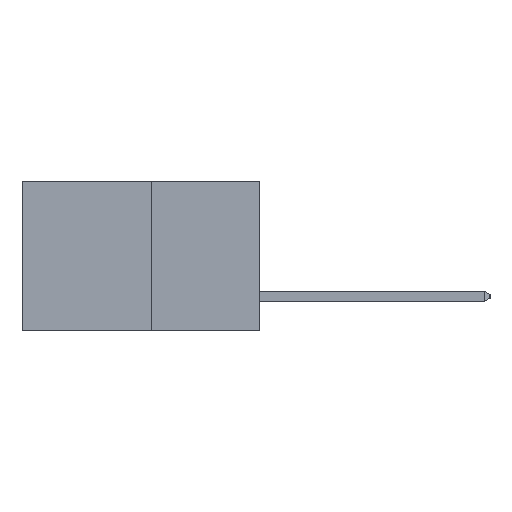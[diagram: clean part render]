
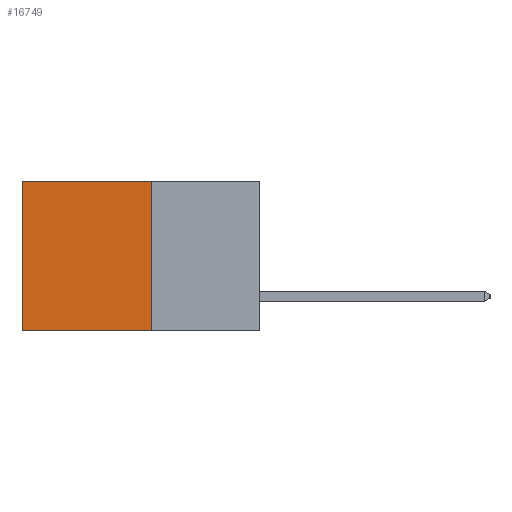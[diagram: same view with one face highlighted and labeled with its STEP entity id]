
A CAD part, left-side view. The second image highlights one B-rep face of the part: STEP entity #16749.
In plain terms, the highlighted planar face has unit normal (-1, 0, 0).
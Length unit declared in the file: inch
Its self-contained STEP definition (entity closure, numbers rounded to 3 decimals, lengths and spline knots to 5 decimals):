
#731 = EDGE_CURVE ( 'NONE', #30358, #21809, #27462, .T. ) ;
#1833 = CARTESIAN_POINT ( 'NONE',  ( 0.277, 0.59, 0. ) ) ;
#1855 = VECTOR ( 'NONE', #16808, 39.37008 ) ;
#1950 = ORIENTED_EDGE ( 'NONE', *, *, #9911, .T. ) ;
#4572 = ORIENTED_EDGE ( 'NONE', *, *, #23207, .T. ) ;
#6554 = CARTESIAN_POINT ( 'NONE',  ( 0.277, 0.27, -0.37 ) ) ;
#7185 = ORIENTED_EDGE ( 'NONE', *, *, #731, .F. ) ;
#7354 = VECTOR ( 'NONE', #25983, 39.37008 ) ;
#8844 = EDGE_CURVE ( 'NONE', #23797, #30358, #12728, .T. ) ;
#8888 = CARTESIAN_POINT ( 'NONE',  ( 0.277, 0.27, 0. ) ) ;
#9094 = PLANE ( 'NONE',  #20618 ) ;
#9911 = EDGE_CURVE ( 'NONE', #22084, #21809, #14952, .T. ) ;
#11354 = FACE_OUTER_BOUND ( 'NONE', #27875, .T. ) ;
#12728 = LINE ( 'NONE', #6554, #17836 ) ;
#12900 = CARTESIAN_POINT ( 'NONE',  ( 0.277, 0.27, -0.37 ) ) ;
#13254 = VECTOR ( 'NONE', #21573, 39.37008 ) ;
#13671 = CARTESIAN_POINT ( 'NONE',  ( 0.277, 0.59, -0.37 ) ) ;
#14195 = DIRECTION ( 'NONE',  ( 0., 0., -1. ) ) ;
#14256 = CARTESIAN_POINT ( 'NONE',  ( 0.277, 0.27, 0. ) ) ;
#14952 = LINE ( 'NONE', #23410, #7354 ) ;
#15652 = LINE ( 'NONE', #14256, #1855 ) ;
#16749 = ADVANCED_FACE ( 'NONE', ( #11354 ), #9094, .F. ) ;
#16808 = DIRECTION ( 'NONE',  ( 0., 1., 0. ) ) ;
#17836 = VECTOR ( 'NONE', #26914, 39.37008 ) ;
#18593 = CARTESIAN_POINT ( 'NONE',  ( 0.277, 0.27, -0.37 ) ) ;
#20618 = AXIS2_PLACEMENT_3D ( 'NONE', #26826, #29241, #14195 ) ;
#20631 = ORIENTED_EDGE ( 'NONE', *, *, #8844, .F. ) ;
#21573 = DIRECTION ( 'NONE',  ( 0., 1., 0. ) ) ;
#21809 = VERTEX_POINT ( 'NONE', #13671 ) ;
#22084 = VERTEX_POINT ( 'NONE', #1833 ) ;
#23207 = EDGE_CURVE ( 'NONE', #23797, #22084, #15652, .T. ) ;
#23410 = CARTESIAN_POINT ( 'NONE',  ( 0.277, 0.59, -0.37 ) ) ;
#23797 = VERTEX_POINT ( 'NONE', #8888 ) ;
#25983 = DIRECTION ( 'NONE',  ( 0., 0., -1. ) ) ;
#26826 = CARTESIAN_POINT ( 'NONE',  ( 0.277, 0.27, -0.37 ) ) ;
#26914 = DIRECTION ( 'NONE',  ( 0., 0., -1. ) ) ;
#27462 = LINE ( 'NONE', #12900, #13254 ) ;
#27875 = EDGE_LOOP ( 'NONE', ( #1950, #7185, #20631, #4572 ) ) ;
#29241 = DIRECTION ( 'NONE',  ( 1., 0., 0. ) ) ;
#30358 = VERTEX_POINT ( 'NONE', #18593 ) ;
